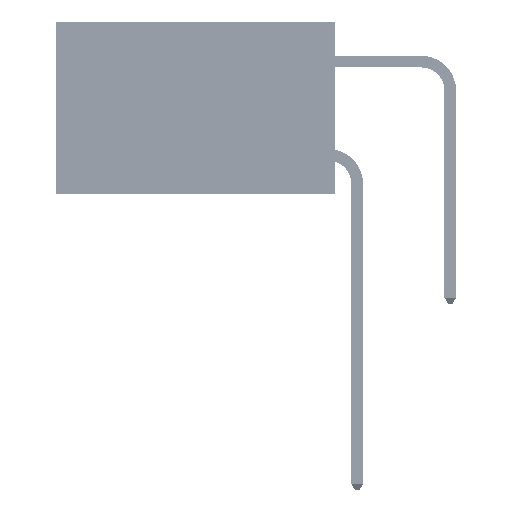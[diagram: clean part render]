
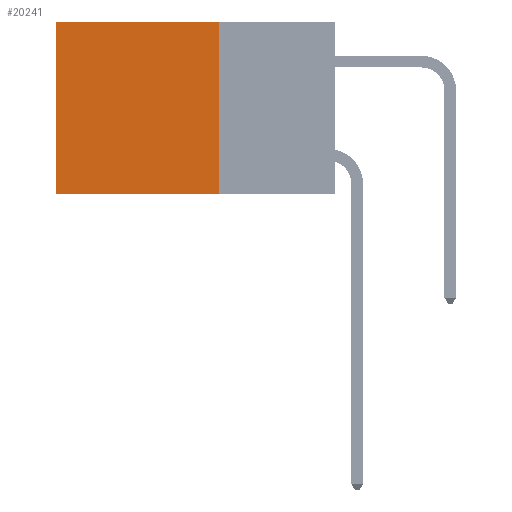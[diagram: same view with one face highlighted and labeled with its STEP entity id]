
A CAD part, left-side view. The second image highlights one B-rep face of the part: STEP entity #20241.
In plain terms, the highlighted planar face has unit normal (-1, 0, 0).
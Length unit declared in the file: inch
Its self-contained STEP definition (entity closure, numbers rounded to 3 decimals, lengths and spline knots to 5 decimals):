
#529 = VECTOR ( 'NONE', #43441, 39.37008 ) ;
#1694 = LINE ( 'NONE', #36272, #529 ) ;
#3335 = DIRECTION ( 'NONE',  ( 1., 0., 0. ) ) ;
#4024 = VECTOR ( 'NONE', #45921, 39.37008 ) ;
#4240 = DIRECTION ( 'NONE',  ( 0., 1., 0. ) ) ;
#5209 = LINE ( 'NONE', #13479, #4024 ) ;
#8867 = CARTESIAN_POINT ( 'NONE',  ( 0.2875, 0.25, -0.37 ) ) ;
#10748 = VERTEX_POINT ( 'NONE', #27090 ) ;
#12561 = VERTEX_POINT ( 'NONE', #19152 ) ;
#13479 = CARTESIAN_POINT ( 'NONE',  ( 0.2875, 0.25, 0. ) ) ;
#14278 = CARTESIAN_POINT ( 'NONE',  ( 0.2875, 0.25, 0. ) ) ;
#19152 = CARTESIAN_POINT ( 'NONE',  ( 0.2875, 0.6, 0. ) ) ;
#20226 = EDGE_LOOP ( 'NONE', ( #37039, #20827, #42390, #20731 ) ) ;
#20241 = ADVANCED_FACE ( 'NONE', ( #46010 ), #43129, .F. ) ;
#20731 = ORIENTED_EDGE ( 'NONE', *, *, #38033, .T. ) ;
#20827 = ORIENTED_EDGE ( 'NONE', *, *, #43785, .F. ) ;
#23111 = VECTOR ( 'NONE', #23401, 39.37008 ) ;
#23401 = DIRECTION ( 'NONE',  ( 0., 1., 0. ) ) ;
#24237 = LINE ( 'NONE', #8867, #23111 ) ;
#24857 = VERTEX_POINT ( 'NONE', #35371 ) ;
#27090 = CARTESIAN_POINT ( 'NONE',  ( 0.2875, 0.25, 0. ) ) ;
#27797 = LINE ( 'NONE', #40564, #30086 ) ;
#28911 = DIRECTION ( 'NONE',  ( 0., 0., -1. ) ) ;
#30086 = VECTOR ( 'NONE', #4240, 39.37008 ) ;
#30782 = EDGE_CURVE ( 'NONE', #10748, #32662, #5209, .T. ) ;
#32662 = VERTEX_POINT ( 'NONE', #42123 ) ;
#35371 = CARTESIAN_POINT ( 'NONE',  ( 0.2875, 0.6, -0.37 ) ) ;
#36272 = CARTESIAN_POINT ( 'NONE',  ( 0.2875, 0.6, 0. ) ) ;
#37039 = ORIENTED_EDGE ( 'NONE', *, *, #46041, .T. ) ;
#38033 = EDGE_CURVE ( 'NONE', #10748, #12561, #27797, .T. ) ;
#40564 = CARTESIAN_POINT ( 'NONE',  ( 0.2875, 0.25, 0. ) ) ;
#41104 = AXIS2_PLACEMENT_3D ( 'NONE', #14278, #3335, #28911 ) ;
#42123 = CARTESIAN_POINT ( 'NONE',  ( 0.2875, 0.25, -0.37 ) ) ;
#42390 = ORIENTED_EDGE ( 'NONE', *, *, #30782, .F. ) ;
#43129 = PLANE ( 'NONE',  #41104 ) ;
#43441 = DIRECTION ( 'NONE',  ( 0., 0., -1. ) ) ;
#43785 = EDGE_CURVE ( 'NONE', #32662, #24857, #24237, .T. ) ;
#45921 = DIRECTION ( 'NONE',  ( 0., 0., -1. ) ) ;
#46010 = FACE_OUTER_BOUND ( 'NONE', #20226, .T. ) ;
#46041 = EDGE_CURVE ( 'NONE', #12561, #24857, #1694, .T. ) ;
